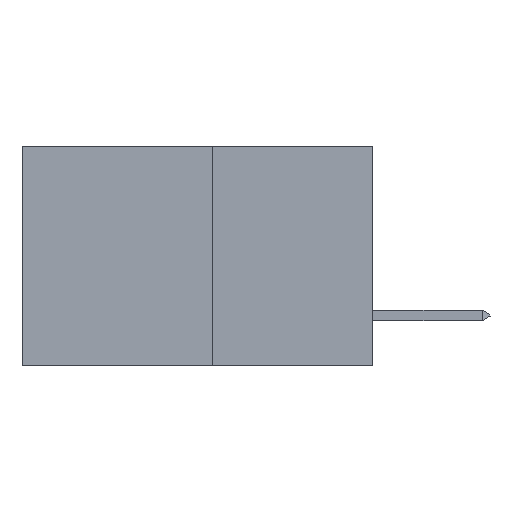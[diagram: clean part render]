
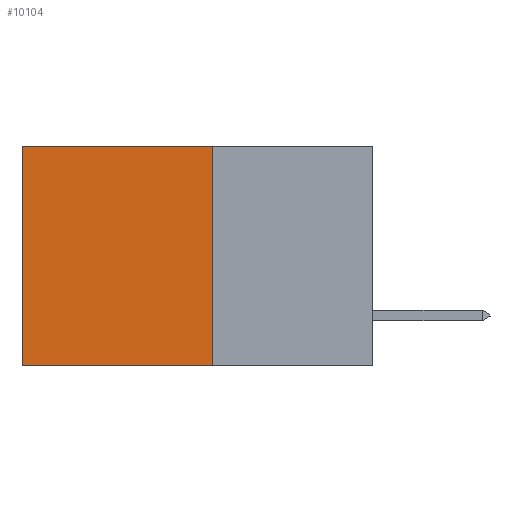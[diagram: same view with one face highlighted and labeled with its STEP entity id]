
A CAD part, left-side view. The second image highlights one B-rep face of the part: STEP entity #10104.
In plain terms, the highlighted planar face has unit normal (-1, 0, 0).
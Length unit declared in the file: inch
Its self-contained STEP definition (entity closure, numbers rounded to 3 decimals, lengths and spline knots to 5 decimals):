
#821 = VERTEX_POINT ( 'NONE', #7386 ) ;
#933 = DIRECTION ( 'NONE',  ( 0., 0., -1. ) ) ;
#1919 = CARTESIAN_POINT ( 'NONE',  ( 0.277, 0.59, -0.37 ) ) ;
#2596 = ORIENTED_EDGE ( 'NONE', *, *, #12885, .T. ) ;
#2632 = EDGE_CURVE ( 'NONE', #821, #5434, #7425, .T. ) ;
#3486 = LINE ( 'NONE', #4222, #12426 ) ;
#3678 = VECTOR ( 'NONE', #6953, 39.37008 ) ;
#4002 = CARTESIAN_POINT ( 'NONE',  ( 0.277, 0.59, -0.37 ) ) ;
#4222 = CARTESIAN_POINT ( 'NONE',  ( 0.277, 0.27, -0.37 ) ) ;
#4357 = DIRECTION ( 'NONE',  ( 0., 0., -1. ) ) ;
#4900 = CARTESIAN_POINT ( 'NONE',  ( 0.277, 0.27, -0.37 ) ) ;
#5070 = VECTOR ( 'NONE', #5610, 39.37008 ) ;
#5434 = VERTEX_POINT ( 'NONE', #1919 ) ;
#5610 = DIRECTION ( 'NONE',  ( 0., 1., 0. ) ) ;
#5644 = ORIENTED_EDGE ( 'NONE', *, *, #9467, .F. ) ;
#5654 = AXIS2_PLACEMENT_3D ( 'NONE', #8981, #7875, #933 ) ;
#6677 = FACE_OUTER_BOUND ( 'NONE', #11586, .T. ) ;
#6953 = DIRECTION ( 'NONE',  ( 0., 1., 0. ) ) ;
#6974 = CARTESIAN_POINT ( 'NONE',  ( 0.277, 0.27, -0.37 ) ) ;
#7386 = CARTESIAN_POINT ( 'NONE',  ( 0.277, 0.59, 0. ) ) ;
#7425 = LINE ( 'NONE', #4002, #12629 ) ;
#7875 = DIRECTION ( 'NONE',  ( 1., 0., 0. ) ) ;
#8562 = ORIENTED_EDGE ( 'NONE', *, *, #9229, .F. ) ;
#8981 = CARTESIAN_POINT ( 'NONE',  ( 0.277, 0.27, -0.37 ) ) ;
#9229 = EDGE_CURVE ( 'NONE', #11574, #5434, #12940, .T. ) ;
#9467 = EDGE_CURVE ( 'NONE', #10089, #11574, #3486, .T. ) ;
#10036 = CARTESIAN_POINT ( 'NONE',  ( 0.277, 0.27, 0. ) ) ;
#10089 = VERTEX_POINT ( 'NONE', #10036 ) ;
#10104 = ADVANCED_FACE ( 'NONE', ( #6677 ), #12282, .F. ) ;
#11343 = LINE ( 'NONE', #14304, #5070 ) ;
#11574 = VERTEX_POINT ( 'NONE', #4900 ) ;
#11586 = EDGE_LOOP ( 'NONE', ( #13658, #8562, #5644, #2596 ) ) ;
#12184 = DIRECTION ( 'NONE',  ( 0., 0., -1. ) ) ;
#12282 = PLANE ( 'NONE',  #5654 ) ;
#12426 = VECTOR ( 'NONE', #4357, 39.37008 ) ;
#12629 = VECTOR ( 'NONE', #12184, 39.37008 ) ;
#12885 = EDGE_CURVE ( 'NONE', #10089, #821, #11343, .T. ) ;
#12940 = LINE ( 'NONE', #6974, #3678 ) ;
#13658 = ORIENTED_EDGE ( 'NONE', *, *, #2632, .T. ) ;
#14304 = CARTESIAN_POINT ( 'NONE',  ( 0.277, 0.27, 0. ) ) ;
